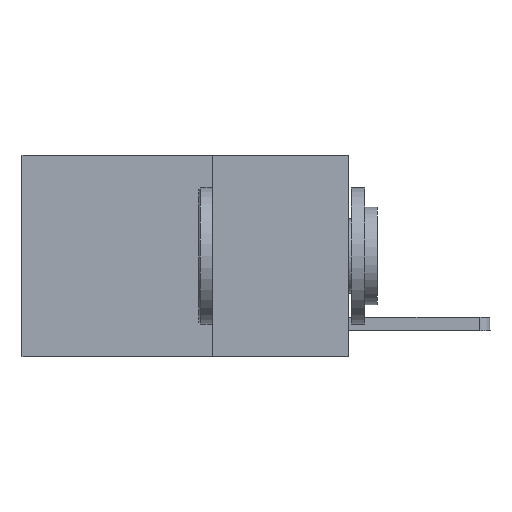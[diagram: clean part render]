
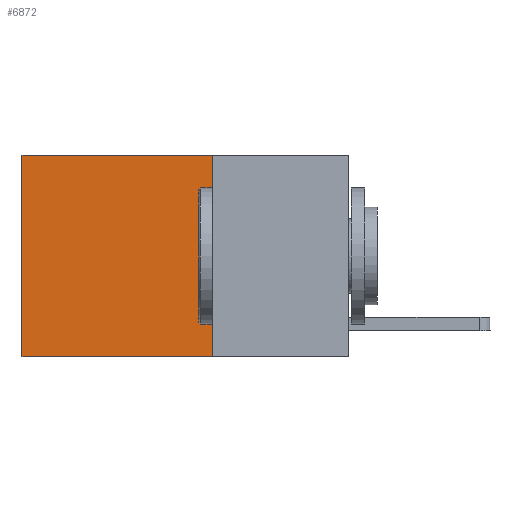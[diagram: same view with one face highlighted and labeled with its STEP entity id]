
A CAD part, left-side view. The second image highlights one B-rep face of the part: STEP entity #6872.
In plain terms, the highlighted planar face has unit normal (-1, 0, 0).
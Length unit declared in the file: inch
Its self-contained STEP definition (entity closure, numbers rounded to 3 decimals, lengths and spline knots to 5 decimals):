
#280 = LINE ( 'NONE', #5914, #4225 ) ;
#335 = CARTESIAN_POINT ( 'NONE',  ( 0.2625, 0.25, 0. ) ) ;
#382 = VERTEX_POINT ( 'NONE', #5491 ) ;
#698 = CARTESIAN_POINT ( 'NONE',  ( 0.2625, 0.6, -0.37 ) ) ;
#962 = VERTEX_POINT ( 'NONE', #335 ) ;
#1020 = ORIENTED_EDGE ( 'NONE', *, *, #8678, .T. ) ;
#1156 = VERTEX_POINT ( 'NONE', #698 ) ;
#1470 = ORIENTED_EDGE ( 'NONE', *, *, #3310, .T. ) ;
#1716 = CARTESIAN_POINT ( 'NONE',  ( 0.2625, 0.25, -0.37 ) ) ;
#1878 = VECTOR ( 'NONE', #8554, 39.37008 ) ;
#2007 = DIRECTION ( 'NONE',  ( 0., 0., -1. ) ) ;
#2095 = AXIS2_PLACEMENT_3D ( 'NONE', #6476, #3795, #5140 ) ;
#2389 = EDGE_CURVE ( 'NONE', #962, #382, #3393, .T. ) ;
#3310 = EDGE_CURVE ( 'NONE', #5343, #1156, #4189, .T. ) ;
#3393 = LINE ( 'NONE', #4691, #7640 ) ;
#3585 = ORIENTED_EDGE ( 'NONE', *, *, #2389, .F. ) ;
#3652 = PLANE ( 'NONE',  #2095 ) ;
#3795 = DIRECTION ( 'NONE',  ( 1., 0., 0. ) ) ;
#3986 = ORIENTED_EDGE ( 'NONE', *, *, #6961, .F. ) ;
#4189 = LINE ( 'NONE', #6998, #1878 ) ;
#4225 = VECTOR ( 'NONE', #8703, 39.37008 ) ;
#4278 = EDGE_LOOP ( 'NONE', ( #1470, #3986, #3585, #1020 ) ) ;
#4666 = LINE ( 'NONE', #1716, #5939 ) ;
#4691 = CARTESIAN_POINT ( 'NONE',  ( 0.2625, 0.25, 0. ) ) ;
#5140 = DIRECTION ( 'NONE',  ( 0., 0., -1. ) ) ;
#5343 = VERTEX_POINT ( 'NONE', #7612 ) ;
#5491 = CARTESIAN_POINT ( 'NONE',  ( 0.2625, 0.25, -0.37 ) ) ;
#5914 = CARTESIAN_POINT ( 'NONE',  ( 0.2625, 0.25, 0. ) ) ;
#5939 = VECTOR ( 'NONE', #7389, 39.37008 ) ;
#6476 = CARTESIAN_POINT ( 'NONE',  ( 0.2625, 0.25, 0. ) ) ;
#6872 = ADVANCED_FACE ( 'NONE', ( #7150 ), #3652, .F. ) ;
#6961 = EDGE_CURVE ( 'NONE', #382, #1156, #4666, .T. ) ;
#6998 = CARTESIAN_POINT ( 'NONE',  ( 0.2625, 0.6, 0. ) ) ;
#7150 = FACE_OUTER_BOUND ( 'NONE', #4278, .T. ) ;
#7389 = DIRECTION ( 'NONE',  ( 0., 1., 0. ) ) ;
#7612 = CARTESIAN_POINT ( 'NONE',  ( 0.2625, 0.6, 0. ) ) ;
#7640 = VECTOR ( 'NONE', #2007, 39.37008 ) ;
#8554 = DIRECTION ( 'NONE',  ( 0., 0., -1. ) ) ;
#8678 = EDGE_CURVE ( 'NONE', #962, #5343, #280, .T. ) ;
#8703 = DIRECTION ( 'NONE',  ( 0., 1., 0. ) ) ;
